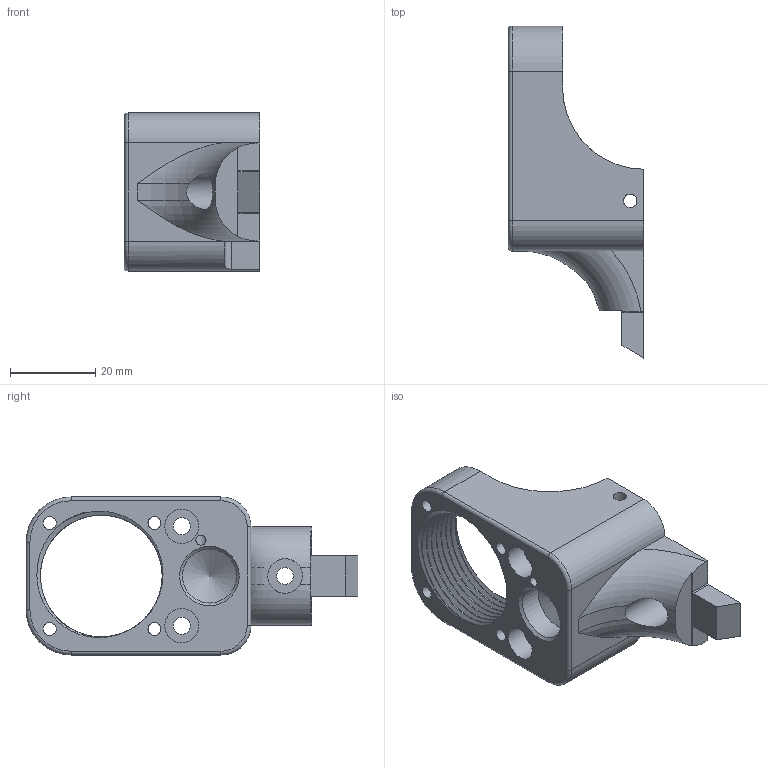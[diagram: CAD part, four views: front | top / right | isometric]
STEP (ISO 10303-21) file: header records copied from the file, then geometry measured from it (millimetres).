
FILE_DESCRIPTION(/* description */ (' '),/* implementation_level */ '2;1');
FILE_NAME(/* name */ 'Buffer Tower.stp',/* time_stamp */ '2019-07-22T21:10:59-05:00',/* author */ ('johne'),/* organization */ (' '),/* preprocessor_version */ 'ST-DEVELOPER v16.13',/* originating_system */ 'Autodesk Inventor 2018',/* authorisation */ ' ');
FILE_SCHEMA (('AUTOMOTIVE_DESIGN { 1 0 10303 214 3 1 1 }'));
Length unit declared in the file: inch
Products named in the file (1): Buffer Tower
Bounding box: 31.83 x 77.95 x 37.13 mm (x, y, z)
Volume: 28677.8 mm3; surface area: 12984.1 mm2
Topology: 1 solids, 1 shells, 111 faces, 314 edges, 205 vertices
Faces by surface type: cylinder 47, bspline 28, plane 25, torus 8, cone 3
Full cylindrical faces by diameter (mm): 2.388 x1, 3.023 x4, 3.175 x2, 3.937 x3, 6.477 x1, 8.001 x2, 8.128 x1, 12.7 x1
Entity records: 5384 total; most frequent: CARTESIAN_POINT 2766, ORIENTED_EDGE 576, DIRECTION 473, EDGE_CURVE 288, AXIS2_PLACEMENT_3D 202, VERTEX_POINT 197, EDGE_LOOP 151, FACE_OUTER_BOUND 111
